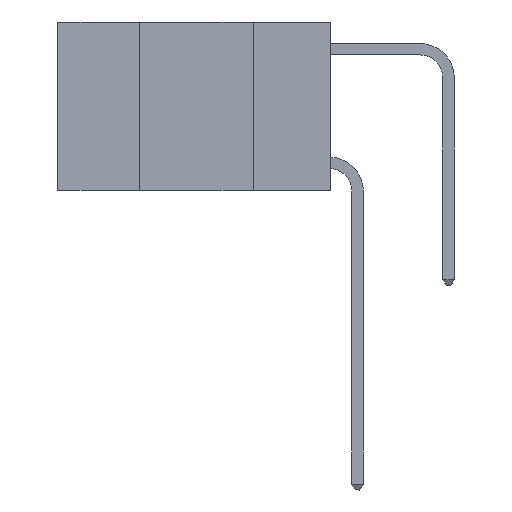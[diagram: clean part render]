
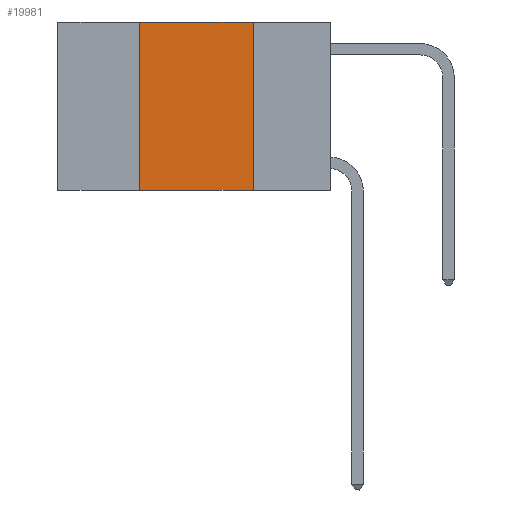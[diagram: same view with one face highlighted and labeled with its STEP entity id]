
A CAD part, left-side view. The second image highlights one B-rep face of the part: STEP entity #19981.
In plain terms, the highlighted planar face has unit normal (-1, 0, 0).
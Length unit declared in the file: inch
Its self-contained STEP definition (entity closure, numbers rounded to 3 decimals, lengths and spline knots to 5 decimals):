
#379 = CARTESIAN_POINT ( 'NONE',  ( 0., 0.42, 0. ) ) ;
#1439 = CARTESIAN_POINT ( 'NONE',  ( 0., 0.42, -0.37 ) ) ;
#1985 = VERTEX_POINT ( 'NONE', #29992 ) ;
#2402 = DIRECTION ( 'NONE',  ( 0., -1., 0. ) ) ;
#2408 = EDGE_CURVE ( 'NONE', #21221, #22262, #16920, .T. ) ;
#3134 = EDGE_CURVE ( 'NONE', #7992, #1985, #11137, .T. ) ;
#6455 = ORIENTED_EDGE ( 'NONE', *, *, #2408, .F. ) ;
#6925 = CARTESIAN_POINT ( 'NONE',  ( 0., 0.6, 0. ) ) ;
#7442 = DIRECTION ( 'NONE',  ( 1., 0., 0. ) ) ;
#7992 = VERTEX_POINT ( 'NONE', #21295 ) ;
#9845 = VECTOR ( 'NONE', #25638, 39.37008 ) ;
#10136 = DIRECTION ( 'NONE',  ( 0., 0., 1. ) ) ;
#11137 = LINE ( 'NONE', #16353, #30179 ) ;
#12957 = ORIENTED_EDGE ( 'NONE', *, *, #27101, .F. ) ;
#14085 = ORIENTED_EDGE ( 'NONE', *, *, #3134, .F. ) ;
#14940 = VECTOR ( 'NONE', #2402, 39.37008 ) ;
#15283 = VECTOR ( 'NONE', #10136, 39.37008 ) ;
#16353 = CARTESIAN_POINT ( 'NONE',  ( 0., 0.17, 0. ) ) ;
#16920 = LINE ( 'NONE', #26229, #15283 ) ;
#19183 = CARTESIAN_POINT ( 'NONE',  ( 0., 0.6, 0. ) ) ;
#19338 = DIRECTION ( 'NONE',  ( 0., 0., -1. ) ) ;
#19637 = PLANE ( 'NONE',  #20403 ) ;
#19742 = EDGE_LOOP ( 'NONE', ( #14085, #12957, #6455, #24459 ) ) ;
#19981 = ADVANCED_FACE ( 'NONE', ( #21946 ), #19637, .F. ) ;
#20403 = AXIS2_PLACEMENT_3D ( 'NONE', #19183, #7442, #19338 ) ;
#21221 = VERTEX_POINT ( 'NONE', #1439 ) ;
#21295 = CARTESIAN_POINT ( 'NONE',  ( 0., 0.17, 0. ) ) ;
#21946 = FACE_OUTER_BOUND ( 'NONE', #19742, .T. ) ;
#22262 = VERTEX_POINT ( 'NONE', #379 ) ;
#23120 = CARTESIAN_POINT ( 'NONE',  ( 0., 0.6, -0.37 ) ) ;
#23579 = LINE ( 'NONE', #23120, #14940 ) ;
#24459 = ORIENTED_EDGE ( 'NONE', *, *, #29837, .T. ) ;
#25638 = DIRECTION ( 'NONE',  ( 0., -1., 0. ) ) ;
#25809 = DIRECTION ( 'NONE',  ( 0., 0., -1. ) ) ;
#25945 = LINE ( 'NONE', #6925, #9845 ) ;
#26229 = CARTESIAN_POINT ( 'NONE',  ( 0., 0.42, 0. ) ) ;
#27101 = EDGE_CURVE ( 'NONE', #22262, #7992, #25945, .T. ) ;
#29837 = EDGE_CURVE ( 'NONE', #21221, #1985, #23579, .T. ) ;
#29992 = CARTESIAN_POINT ( 'NONE',  ( 0., 0.17, -0.37 ) ) ;
#30179 = VECTOR ( 'NONE', #25809, 39.37008 ) ;
